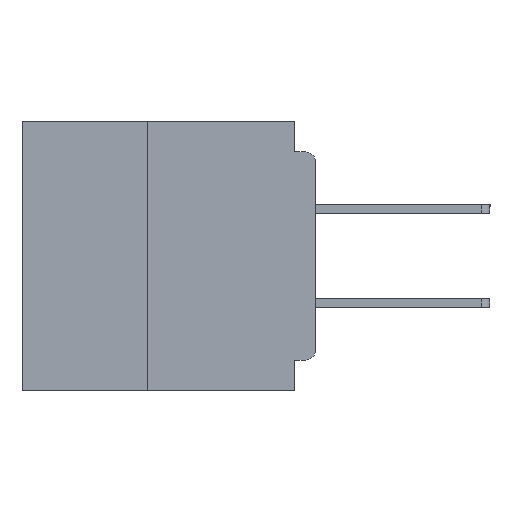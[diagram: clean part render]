
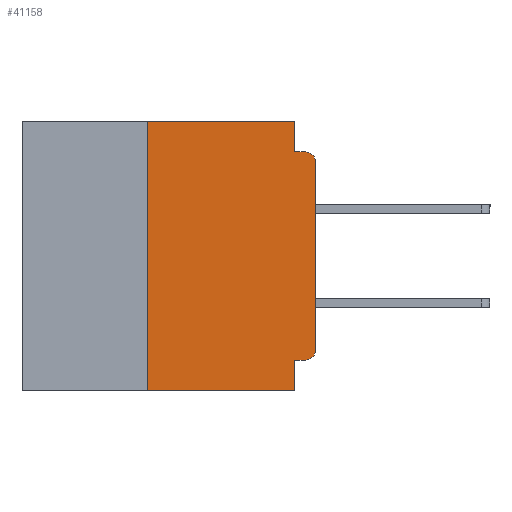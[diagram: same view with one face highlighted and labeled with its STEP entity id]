
A CAD part, left-side view. The second image highlights one B-rep face of the part: STEP entity #41158.
In plain terms, the highlighted planar face has unit normal (-1, 0, 0).
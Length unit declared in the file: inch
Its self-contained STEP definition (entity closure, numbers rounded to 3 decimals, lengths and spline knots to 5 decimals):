
#1267 = VECTOR ( 'NONE', #1572, 39.37008 ) ;
#1572 = DIRECTION ( 'NONE',  ( 0., 0., 1. ) ) ;
#1998 = DIRECTION ( 'NONE',  ( 1., 0., 0. ) ) ;
#2041 = CARTESIAN_POINT ( 'NONE',  ( 0., 0., -0.355 ) ) ;
#2167 = ORIENTED_EDGE ( 'NONE', *, *, #26343, .F. ) ;
#2186 = VECTOR ( 'NONE', #19253, 39.37008 ) ;
#2716 = DIRECTION ( 'NONE',  ( 0., -1., 0. ) ) ;
#4154 = EDGE_CURVE ( 'NONE', #12791, #11370, #24992, .T. ) ;
#5544 = DIRECTION ( 'NONE',  ( 0., 1., 0. ) ) ;
#5643 = LINE ( 'NONE', #23657, #12687 ) ;
#6070 = EDGE_CURVE ( 'NONE', #14621, #36281, #18408, .T. ) ;
#6870 = LINE ( 'NONE', #34261, #41512 ) ;
#7192 = CARTESIAN_POINT ( 'NONE',  ( 0., 0.25, -0.4 ) ) ;
#8117 = CIRCLE ( 'NONE', #32537, 0.015 ) ;
#8302 = CARTESIAN_POINT ( 'NONE',  ( 0., 0.031, -0.4 ) ) ;
#8497 = CARTESIAN_POINT ( 'NONE',  ( 0., 0.031, 0. ) ) ;
#8889 = CIRCLE ( 'NONE', #18335, 0.015 ) ;
#9334 = VERTEX_POINT ( 'NONE', #20868 ) ;
#9887 = EDGE_CURVE ( 'NONE', #25356, #36281, #5643, .T. ) ;
#11370 = VERTEX_POINT ( 'NONE', #27889 ) ;
#12513 = LINE ( 'NONE', #15744, #2186 ) ;
#12687 = VECTOR ( 'NONE', #44325, 39.37008 ) ;
#12791 = VERTEX_POINT ( 'NONE', #8497 ) ;
#14621 = VERTEX_POINT ( 'NONE', #7192 ) ;
#15271 = ORIENTED_EDGE ( 'NONE', *, *, #9887, .F. ) ;
#15744 = CARTESIAN_POINT ( 'NONE',  ( 0., 0., 0. ) ) ;
#16386 = DIRECTION ( 'NONE',  ( -1., 0., 0. ) ) ;
#16460 = VERTEX_POINT ( 'NONE', #20851 ) ;
#17324 = VERTEX_POINT ( 'NONE', #39297 ) ;
#18335 = AXIS2_PLACEMENT_3D ( 'NONE', #37171, #16386, #40588 ) ;
#18408 = LINE ( 'NONE', #41945, #43765 ) ;
#18479 = AXIS2_PLACEMENT_3D ( 'NONE', #33105, #1998, #26209 ) ;
#19167 = DIRECTION ( 'NONE',  ( -1., 0., 0. ) ) ;
#19253 = DIRECTION ( 'NONE',  ( 0., 0., 1. ) ) ;
#19268 = CARTESIAN_POINT ( 'NONE',  ( 0., 0.031, -0.355 ) ) ;
#20851 = CARTESIAN_POINT ( 'NONE',  ( 0., 0.015, -0.355 ) ) ;
#20868 = CARTESIAN_POINT ( 'NONE',  ( 0., 0., -0.34 ) ) ;
#21318 = ORIENTED_EDGE ( 'NONE', *, *, #42374, .F. ) ;
#21894 = ORIENTED_EDGE ( 'NONE', *, *, #41065, .F. ) ;
#22006 = EDGE_CURVE ( 'NONE', #17324, #22101, #8889, .T. ) ;
#22101 = VERTEX_POINT ( 'NONE', #27273 ) ;
#23657 = CARTESIAN_POINT ( 'NONE',  ( 0., 0.031, -0.4 ) ) ;
#24245 = LINE ( 'NONE', #2041, #41555 ) ;
#24541 = FACE_OUTER_BOUND ( 'NONE', #28333, .T. ) ;
#24992 = LINE ( 'NONE', #40454, #42275 ) ;
#25356 = VERTEX_POINT ( 'NONE', #19268 ) ;
#26209 = DIRECTION ( 'NONE',  ( 0., 0., -1. ) ) ;
#26343 = EDGE_CURVE ( 'NONE', #11370, #22101, #6870, .T. ) ;
#27273 = CARTESIAN_POINT ( 'NONE',  ( 0., 0.015, -0.045 ) ) ;
#27436 = VERTEX_POINT ( 'NONE', #29592 ) ;
#27786 = ORIENTED_EDGE ( 'NONE', *, *, #4154, .F. ) ;
#27832 = LINE ( 'NONE', #42978, #1267 ) ;
#27889 = CARTESIAN_POINT ( 'NONE',  ( 0., 0.031, -0.045 ) ) ;
#28333 = EDGE_LOOP ( 'NONE', ( #32906, #39859, #2167, #27786, #33413, #21894, #31090, #15271, #21318, #40066 ) ) ;
#29592 = CARTESIAN_POINT ( 'NONE',  ( 0., 0.25, 0. ) ) ;
#30123 = EDGE_CURVE ( 'NONE', #27436, #12791, #41360, .T. ) ;
#31090 = ORIENTED_EDGE ( 'NONE', *, *, #6070, .T. ) ;
#32029 = EDGE_CURVE ( 'NONE', #9334, #17324, #12513, .T. ) ;
#32235 = VECTOR ( 'NONE', #2716, 39.37008 ) ;
#32537 = AXIS2_PLACEMENT_3D ( 'NONE', #39909, #19167, #43299 ) ;
#32906 = ORIENTED_EDGE ( 'NONE', *, *, #32029, .T. ) ;
#33105 = CARTESIAN_POINT ( 'NONE',  ( 0., 0.437, 0. ) ) ;
#33241 = EDGE_CURVE ( 'NONE', #16460, #9334, #8117, .T. ) ;
#33413 = ORIENTED_EDGE ( 'NONE', *, *, #30123, .F. ) ;
#34261 = CARTESIAN_POINT ( 'NONE',  ( 0., 0., -0.045 ) ) ;
#36281 = VERTEX_POINT ( 'NONE', #8302 ) ;
#37171 = CARTESIAN_POINT ( 'NONE',  ( 0., 0.015, -0.06 ) ) ;
#37710 = DIRECTION ( 'NONE',  ( 0., -1., 0. ) ) ;
#39297 = CARTESIAN_POINT ( 'NONE',  ( 0., 0., -0.06 ) ) ;
#39859 = ORIENTED_EDGE ( 'NONE', *, *, #22006, .T. ) ;
#39909 = CARTESIAN_POINT ( 'NONE',  ( 0., 0.015, -0.34 ) ) ;
#40010 = PLANE ( 'NONE',  #18479 ) ;
#40066 = ORIENTED_EDGE ( 'NONE', *, *, #33241, .T. ) ;
#40363 = DIRECTION ( 'NONE',  ( 0., 0., -1. ) ) ;
#40454 = CARTESIAN_POINT ( 'NONE',  ( 0., 0.031, 0. ) ) ;
#40588 = DIRECTION ( 'NONE',  ( 0., 0., -1. ) ) ;
#41065 = EDGE_CURVE ( 'NONE', #14621, #27436, #27832, .T. ) ;
#41158 = ADVANCED_FACE ( 'NONE', ( #24541 ), #40010, .F. ) ;
#41360 = LINE ( 'NONE', #44272, #32235 ) ;
#41512 = VECTOR ( 'NONE', #37710, 39.37008 ) ;
#41555 = VECTOR ( 'NONE', #5544, 39.37008 ) ;
#41803 = DIRECTION ( 'NONE',  ( 0., -1., 0. ) ) ;
#41945 = CARTESIAN_POINT ( 'NONE',  ( 0., 0.437, -0.4 ) ) ;
#42275 = VECTOR ( 'NONE', #40363, 39.37008 ) ;
#42374 = EDGE_CURVE ( 'NONE', #16460, #25356, #24245, .T. ) ;
#42978 = CARTESIAN_POINT ( 'NONE',  ( 0., 0.25, -0.4 ) ) ;
#43299 = DIRECTION ( 'NONE',  ( 0., 0., -1. ) ) ;
#43765 = VECTOR ( 'NONE', #41803, 39.37008 ) ;
#44272 = CARTESIAN_POINT ( 'NONE',  ( 0., 0.437, 0. ) ) ;
#44325 = DIRECTION ( 'NONE',  ( 0., 0., -1. ) ) ;
